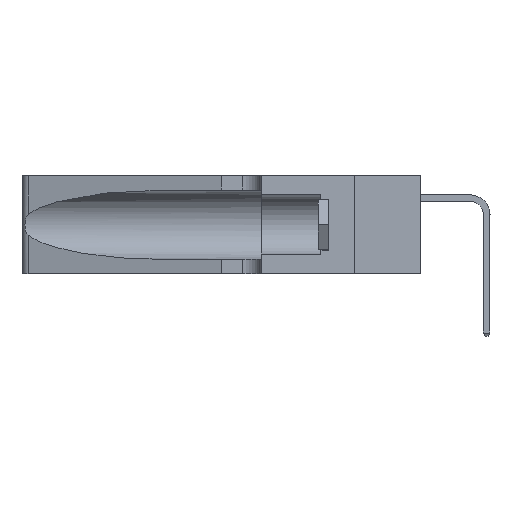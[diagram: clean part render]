
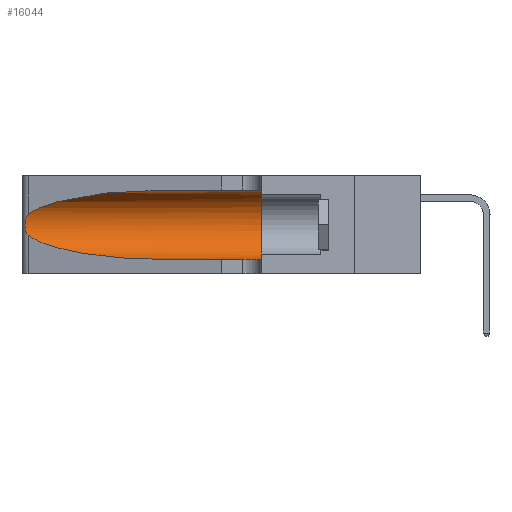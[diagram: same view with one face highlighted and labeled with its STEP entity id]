
A CAD part, left-side view. The second image highlights one B-rep face of the part: STEP entity #16044.
In plain terms, the highlighted cylindrical face has radius 3.308 mm (diameter 6.617 mm), a partial arc.
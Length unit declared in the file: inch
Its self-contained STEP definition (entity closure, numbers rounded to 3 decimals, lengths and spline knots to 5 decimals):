
#579 = DIRECTION ( 'NONE',  ( 0., 0., 1. ) ) ;
#925 = EDGE_CURVE ( 'NONE', #15404, #29260, #31850, .T. ) ;
#1259 = CARTESIAN_POINT ( 'NONE',  ( 0.25487, 1.22718, 0.14631 ) ) ;
#1272 = VECTOR ( 'NONE', #9575, 39.37008 ) ;
#2008 =( BOUNDED_CURVE ( )  B_SPLINE_CURVE ( 3, ( #3959, #31618, #7920, #35578 ),
 .UNSPECIFIED., .F., .F. ) 
 B_SPLINE_CURVE_WITH_KNOTS ( ( 4, 4 ),
 ( 3.44316, 4.71239 ),
 .UNSPECIFIED. ) 
 CURVE ( )  GEOMETRIC_REPRESENTATION_ITEM ( )  RATIONAL_B_SPLINE_CURVE ( ( 1., 0.87, 0.87, 1. ) ) 
 REPRESENTATION_ITEM ( '' )  );
#3440 = VERTEX_POINT ( 'NONE', #18220 ) ;
#3870 = VERTEX_POINT ( 'NONE', #36536 ) ;
#3959 = CARTESIAN_POINT ( 'NONE',  ( 0.25487, 1.22718, 0.14631 ) ) ;
#4678 = AXIS2_PLACEMENT_3D ( 'NONE', #47869, #24291, #579 ) ;
#4697 = EDGE_CURVE ( 'NONE', #25407, #28404, #45869, .T. ) ;
#4754 = CARTESIAN_POINT ( 'NONE',  ( 0.1305, 0.72297, 0.31525 ) ) ;
#4889 = CARTESIAN_POINT ( 'NONE',  ( 0.25487, 1.22718, 0.22369 ) ) ;
#5054 = CARTESIAN_POINT ( 'NONE',  ( 0.25639, 1.23184, 0.21858 ) ) ;
#5131 = DIRECTION ( 'NONE',  ( 0., -1., 0. ) ) ;
#5809 = EDGE_CURVE ( 'NONE', #28404, #3870, #21811, .T. ) ;
#6198 = CARTESIAN_POINT ( 'NONE',  ( 0.1305, 0.72297, 0.31525 ) ) ;
#7046 = EDGE_CURVE ( 'NONE', #3440, #29260, #23981, .T. ) ;
#7920 = CARTESIAN_POINT ( 'NONE',  ( 0.18966, 0.96281, 0.05475 ) ) ;
#9019 = CARTESIAN_POINT ( 'NONE',  ( 0.25854, 1.2359, 0.20912 ) ) ;
#9575 = DIRECTION ( 'NONE',  ( 0., -1., 0. ) ) ;
#11795 = LINE ( 'NONE', #21336, #1272 ) ;
#13010 = CARTESIAN_POINT ( 'NONE',  ( 0.26075, 1.23896, 0.19203 ) ) ;
#14318 = EDGE_LOOP ( 'NONE', ( #35962, #25217, #32034, #24907, #19553, #16397 ) ) ;
#15404 = VERTEX_POINT ( 'NONE', #46430 ) ;
#15804 = CARTESIAN_POINT ( 'NONE',  ( 0.1305, 0.35, 0.05475 ) ) ;
#16044 = ADVANCED_FACE ( 'NONE', ( #35474 ), #34239, .F. ) ;
#16397 = ORIENTED_EDGE ( 'NONE', *, *, #25547, .F. ) ;
#16965 = CARTESIAN_POINT ( 'NONE',  ( 0.26017, 1.23833, 0.17102 ) ) ;
#18220 = CARTESIAN_POINT ( 'NONE',  ( 0.1305, 0.35, 0.31525 ) ) ;
#19439 = CARTESIAN_POINT ( 'NONE',  ( 0.1305, 1.61858, 0.185 ) ) ;
#19553 = ORIENTED_EDGE ( 'NONE', *, *, #7046, .F. ) ;
#20956 = CARTESIAN_POINT ( 'NONE',  ( 0.25789, 1.23486, 0.15765 ) ) ;
#21336 = CARTESIAN_POINT ( 'NONE',  ( 0.1305, 1.61858, 0.31525 ) ) ;
#21811 = B_SPLINE_CURVE_WITH_KNOTS ( 'NONE', 3,
 ( #4889, #24794, #5054, #32723, #9019, #36696, #13010, #40676, #16965, #44610, #20956, #48546, #24960, #1259 ),
 .UNSPECIFIED., .F., .F.,
 ( 4, 2, 2, 2, 2, 2, 4 ),
 ( 0., 0.00027, 0.00053, 0.00107, 0.0016, 0.00187, 0.00214 ),
 .UNSPECIFIED. ) ;
#21948 = CARTESIAN_POINT ( 'NONE',  ( 0.2373, 1.15595, 0.28018 ) ) ;
#23981 = CIRCLE ( 'NONE', #4678, 0.13025 ) ;
#24291 = DIRECTION ( 'NONE',  ( 0., 1., 0. ) ) ;
#24794 = CARTESIAN_POINT ( 'NONE',  ( 0.25555, 1.22994, 0.2215 ) ) ;
#24907 = ORIENTED_EDGE ( 'NONE', *, *, #925, .T. ) ;
#24960 = CARTESIAN_POINT ( 'NONE',  ( 0.25555, 1.22993, 0.14849 ) ) ;
#25217 = ORIENTED_EDGE ( 'NONE', *, *, #5809, .T. ) ;
#25407 = VERTEX_POINT ( 'NONE', #4754 ) ;
#25547 = EDGE_CURVE ( 'NONE', #25407, #3440, #11795, .T. ) ;
#25931 = CARTESIAN_POINT ( 'NONE',  ( 0.18966, 0.96281, 0.31525 ) ) ;
#28404 = VERTEX_POINT ( 'NONE', #37523 ) ;
#29260 = VERTEX_POINT ( 'NONE', #15804 ) ;
#31618 = CARTESIAN_POINT ( 'NONE',  ( 0.2373, 1.15595, 0.08982 ) ) ;
#31850 = LINE ( 'NONE', #48468, #41136 ) ;
#32034 = ORIENTED_EDGE ( 'NONE', *, *, #44361, .T. ) ;
#32723 = CARTESIAN_POINT ( 'NONE',  ( 0.25787, 1.23484, 0.2124 ) ) ;
#33843 = CARTESIAN_POINT ( 'NONE',  ( 0.25487, 1.22718, 0.22369 ) ) ;
#34239 = CYLINDRICAL_SURFACE ( 'NONE', #34736, 0.13025 ) ;
#34736 = AXIS2_PLACEMENT_3D ( 'NONE', #19439, #39180, #35185 ) ;
#35185 = DIRECTION ( 'NONE',  ( 0., 0., -1. ) ) ;
#35474 = FACE_OUTER_BOUND ( 'NONE', #14318, .T. ) ;
#35578 = CARTESIAN_POINT ( 'NONE',  ( 0.1305, 0.72297, 0.05475 ) ) ;
#35962 = ORIENTED_EDGE ( 'NONE', *, *, #4697, .T. ) ;
#36536 = CARTESIAN_POINT ( 'NONE',  ( 0.25487, 1.22718, 0.14631 ) ) ;
#36696 = CARTESIAN_POINT ( 'NONE',  ( 0.26018, 1.23835, 0.19895 ) ) ;
#37523 = CARTESIAN_POINT ( 'NONE',  ( 0.25487, 1.22718, 0.22369 ) ) ;
#39180 = DIRECTION ( 'NONE',  ( 0., -1., 0. ) ) ;
#40676 = CARTESIAN_POINT ( 'NONE',  ( 0.26075, 1.23896, 0.178 ) ) ;
#41136 = VECTOR ( 'NONE', #5131, 39.37008 ) ;
#44361 = EDGE_CURVE ( 'NONE', #3870, #15404, #2008, .T. ) ;
#44610 = CARTESIAN_POINT ( 'NONE',  ( 0.25856, 1.23593, 0.16098 ) ) ;
#45869 =( BOUNDED_CURVE ( )  B_SPLINE_CURVE ( 3, ( #6198, #25931, #21948, #33843 ),
 .UNSPECIFIED., .F., .F. ) 
 B_SPLINE_CURVE_WITH_KNOTS ( ( 4, 4 ),
 ( 1.5708, 2.84003 ),
 .UNSPECIFIED. ) 
 CURVE ( )  GEOMETRIC_REPRESENTATION_ITEM ( )  RATIONAL_B_SPLINE_CURVE ( ( 1., 0.87, 0.87, 1. ) ) 
 REPRESENTATION_ITEM ( '' )  );
#46430 = CARTESIAN_POINT ( 'NONE',  ( 0.1305, 0.72297, 0.05475 ) ) ;
#47869 = CARTESIAN_POINT ( 'NONE',  ( 0.1305, 0.35, 0.185 ) ) ;
#48468 = CARTESIAN_POINT ( 'NONE',  ( 0.1305, 1.61858, 0.05475 ) ) ;
#48546 = CARTESIAN_POINT ( 'NONE',  ( 0.25639, 1.23186, 0.15144 ) ) ;
